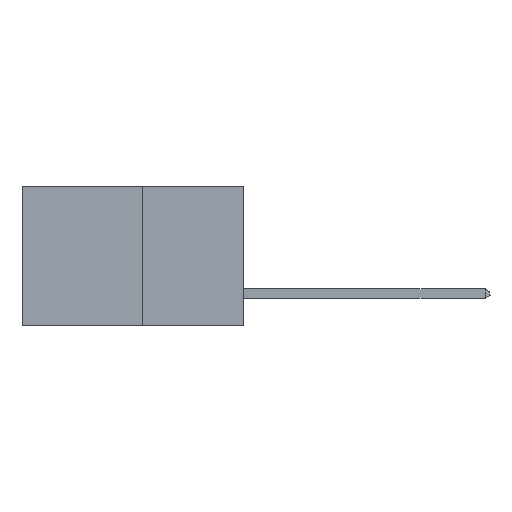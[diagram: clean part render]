
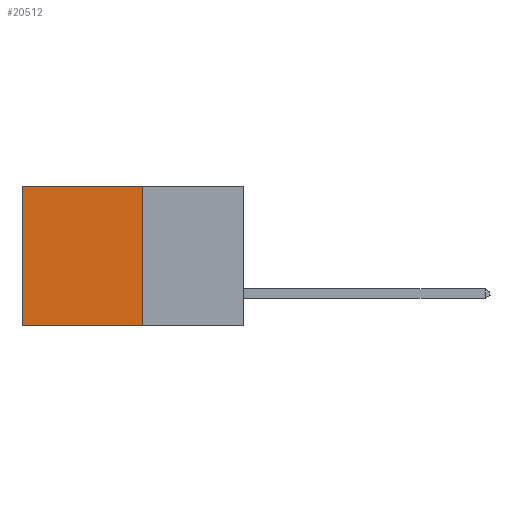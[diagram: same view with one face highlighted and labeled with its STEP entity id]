
A CAD part, left-side view. The second image highlights one B-rep face of the part: STEP entity #20512.
In plain terms, the highlighted planar face has unit normal (-1, 0, 0).
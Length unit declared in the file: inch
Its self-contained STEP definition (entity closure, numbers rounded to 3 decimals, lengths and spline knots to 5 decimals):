
#967 = PLANE ( 'NONE',  #15260 ) ;
#1831 = CARTESIAN_POINT ( 'NONE',  ( 0.277, 0.27, -0.37 ) ) ;
#2617 = DIRECTION ( 'NONE',  ( 0., 0., -1. ) ) ;
#2624 = EDGE_LOOP ( 'NONE', ( #20108, #20311, #20332, #20369 ) ) ;
#2795 = EDGE_CURVE ( 'NONE', #16768, #14716, #14733, .T. ) ;
#3681 = CARTESIAN_POINT ( 'NONE',  ( 0.277, 0.59, -0.37 ) ) ;
#4193 = CARTESIAN_POINT ( 'NONE',  ( 0.277, 0.27, -0.37 ) ) ;
#5205 = CARTESIAN_POINT ( 'NONE',  ( 0.277, 0.27, 0. ) ) ;
#8719 = EDGE_CURVE ( 'NONE', #18233, #14716, #19486, .T. ) ;
#8823 = CARTESIAN_POINT ( 'NONE',  ( 0.277, 0.27, -0.37 ) ) ;
#9158 = LINE ( 'NONE', #1831, #20838 ) ;
#9930 = CARTESIAN_POINT ( 'NONE',  ( 0.277, 0.59, -0.37 ) ) ;
#10266 = VECTOR ( 'NONE', #12117, 39.37008 ) ;
#10494 = VECTOR ( 'NONE', #12906, 39.37008 ) ;
#11519 = DIRECTION ( 'NONE',  ( 0., 0., -1. ) ) ;
#12117 = DIRECTION ( 'NONE',  ( 0., 1., 0. ) ) ;
#12368 = DIRECTION ( 'NONE',  ( 1., 0., 0. ) ) ;
#12906 = DIRECTION ( 'NONE',  ( 0., 1., 0. ) ) ;
#13189 = CARTESIAN_POINT ( 'NONE',  ( 0.277, 0.27, -0.37 ) ) ;
#13818 = FACE_OUTER_BOUND ( 'NONE', #2624, .T. ) ;
#14503 = CARTESIAN_POINT ( 'NONE',  ( 0.277, 0.59, 0. ) ) ;
#14716 = VERTEX_POINT ( 'NONE', #3681 ) ;
#14733 = LINE ( 'NONE', #13189, #10494 ) ;
#15260 = AXIS2_PLACEMENT_3D ( 'NONE', #4193, #12368, #2617 ) ;
#15486 = EDGE_CURVE ( 'NONE', #16643, #18233, #18244, .T. ) ;
#15759 = VECTOR ( 'NONE', #11519, 39.37008 ) ;
#16643 = VERTEX_POINT ( 'NONE', #5205 ) ;
#16768 = VERTEX_POINT ( 'NONE', #8823 ) ;
#17797 = EDGE_CURVE ( 'NONE', #16643, #16768, #9158, .T. ) ;
#17996 = DIRECTION ( 'NONE',  ( 0., 0., -1. ) ) ;
#18233 = VERTEX_POINT ( 'NONE', #14503 ) ;
#18244 = LINE ( 'NONE', #20019, #10266 ) ;
#19486 = LINE ( 'NONE', #9930, #15759 ) ;
#20019 = CARTESIAN_POINT ( 'NONE',  ( 0.277, 0.27, 0. ) ) ;
#20108 = ORIENTED_EDGE ( 'NONE', *, *, #8719, .T. ) ;
#20311 = ORIENTED_EDGE ( 'NONE', *, *, #2795, .F. ) ;
#20332 = ORIENTED_EDGE ( 'NONE', *, *, #17797, .F. ) ;
#20369 = ORIENTED_EDGE ( 'NONE', *, *, #15486, .T. ) ;
#20512 = ADVANCED_FACE ( 'NONE', ( #13818 ), #967, .F. ) ;
#20838 = VECTOR ( 'NONE', #17996, 39.37008 ) ;
